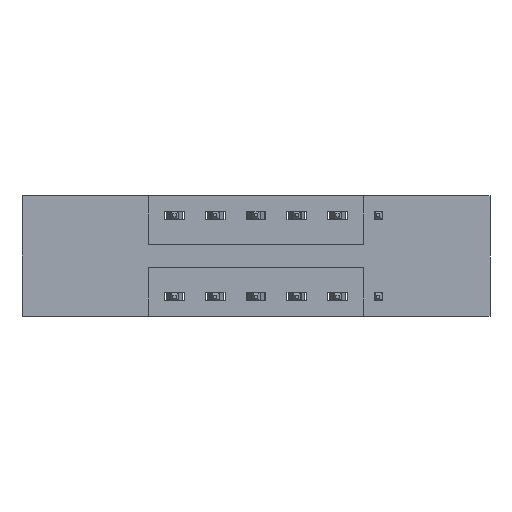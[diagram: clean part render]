
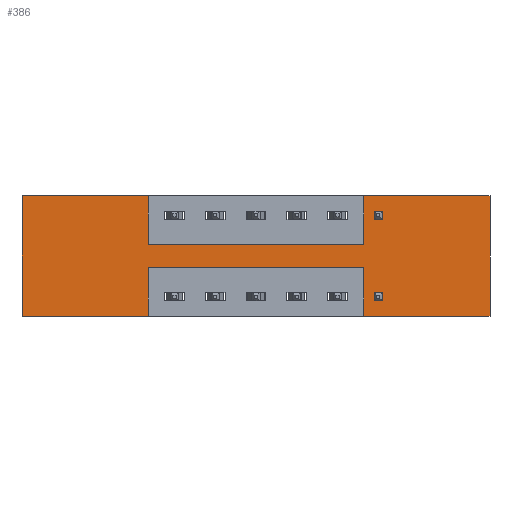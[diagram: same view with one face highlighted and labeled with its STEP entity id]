
A CAD part, front view. The second image highlights one B-rep face of the part: STEP entity #386.
In plain terms, the highlighted planar face has unit normal (0, -1, 0).
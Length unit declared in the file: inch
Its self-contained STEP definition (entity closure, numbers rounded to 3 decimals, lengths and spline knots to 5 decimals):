
#51 = CARTESIAN_POINT ( 'NONE',  ( 0., 0., 0. ) ) ;
#54 = LINE ( 'NONE', #3885, #1753 ) ;
#152 = DIRECTION ( 'NONE',  ( 1., 0., 0. ) ) ;
#193 = CARTESIAN_POINT ( 'NONE',  ( 1.0475, 0., 0. ) ) ;
#250 = VERTEX_POINT ( 'NONE', #798 ) ;
#353 = EDGE_CURVE ( 'NONE', #8071, #6686, #5469, .T. ) ;
#386 = ADVANCED_FACE ( 'NONE', ( #6793 ), #2985, .T. ) ;
#467 = DIRECTION ( 'NONE',  ( 0., -1., 0. ) ) ;
#502 = DIRECTION ( 'NONE',  ( 1., 0., 0. ) ) ;
#661 = CARTESIAN_POINT ( 'NONE',  ( 0., 0., 0. ) ) ;
#690 = VECTOR ( 'NONE', #152, 39.37008 ) ;
#798 = CARTESIAN_POINT ( 'NONE',  ( 0., 0., 0. ) ) ;
#799 = VERTEX_POINT ( 'NONE', #7419 ) ;
#816 = ORIENTED_EDGE ( 'NONE', *, *, #2270, .F. ) ;
#901 = VECTOR ( 'NONE', #8348, 39.37008 ) ;
#942 = VECTOR ( 'NONE', #502, 39.37008 ) ;
#1068 = DIRECTION ( 'NONE',  ( -1., 0., 0. ) ) ;
#1138 = CARTESIAN_POINT ( 'NONE',  ( 1.0475, 0., -0.22 ) ) ;
#1282 = LINE ( 'NONE', #661, #942 ) ;
#1291 = LINE ( 'NONE', #51, #901 ) ;
#1315 = AXIS2_PLACEMENT_3D ( 'NONE', #4908, #467, #3642 ) ;
#1348 = VERTEX_POINT ( 'NONE', #2569 ) ;
#1357 = VERTEX_POINT ( 'NONE', #3238 ) ;
#1665 = LINE ( 'NONE', #4821, #6611 ) ;
#1753 = VECTOR ( 'NONE', #4112, 39.37008 ) ;
#1764 = EDGE_CURVE ( 'NONE', #4762, #2264, #6546, .T. ) ;
#1775 = ORIENTED_EDGE ( 'NONE', *, *, #7255, .F. ) ;
#1805 = DIRECTION ( 'NONE',  ( 0., 0., 1. ) ) ;
#2031 = DIRECTION ( 'NONE',  ( 0., 0., -1. ) ) ;
#2061 = EDGE_CURVE ( 'NONE', #2651, #250, #2506, .T. ) ;
#2093 = DIRECTION ( 'NONE',  ( 0., 0., 1. ) ) ;
#2256 = ORIENTED_EDGE ( 'NONE', *, *, #7544, .F. ) ;
#2264 = VERTEX_POINT ( 'NONE', #7467 ) ;
#2270 = EDGE_CURVE ( 'NONE', #799, #2651, #8138, .T. ) ;
#2292 = LINE ( 'NONE', #6685, #7977 ) ;
#2310 = ORIENTED_EDGE ( 'NONE', *, *, #2061, .F. ) ;
#2506 = LINE ( 'NONE', #8345, #3265 ) ;
#2532 = VECTOR ( 'NONE', #8082, 39.37008 ) ;
#2569 = CARTESIAN_POINT ( 'NONE',  ( 0.3875, 0., -0.22 ) ) ;
#2651 = VERTEX_POINT ( 'NONE', #5196 ) ;
#2677 = LINE ( 'NONE', #5175, #8046 ) ;
#2882 = EDGE_CURVE ( 'NONE', #6908, #6775, #8292, .T. ) ;
#2985 = PLANE ( 'NONE',  #1315 ) ;
#3027 = ORIENTED_EDGE ( 'NONE', *, *, #3664, .F. ) ;
#3066 = ORIENTED_EDGE ( 'NONE', *, *, #3914, .F. ) ;
#3238 = CARTESIAN_POINT ( 'NONE',  ( 0.3875, 0., -0.15 ) ) ;
#3265 = VECTOR ( 'NONE', #3299, 39.37008 ) ;
#3271 = EDGE_CURVE ( 'NONE', #1357, #4762, #3615, .T. ) ;
#3299 = DIRECTION ( 'NONE',  ( 0., 0., 1. ) ) ;
#3323 = CARTESIAN_POINT ( 'NONE',  ( 1.435, 0., -0.37 ) ) ;
#3566 = EDGE_CURVE ( 'NONE', #4511, #1357, #54, .T. ) ;
#3615 = LINE ( 'NONE', #4597, #690 ) ;
#3642 = DIRECTION ( 'NONE',  ( 0., 0., -1. ) ) ;
#3664 = EDGE_CURVE ( 'NONE', #250, #4511, #1282, .T. ) ;
#3788 = CARTESIAN_POINT ( 'NONE',  ( 1.435, 0., 0. ) ) ;
#3800 = VECTOR ( 'NONE', #2093, 39.37008 ) ;
#3885 = CARTESIAN_POINT ( 'NONE',  ( 0.3875, 0., 0. ) ) ;
#3914 = EDGE_CURVE ( 'NONE', #6686, #6908, #1665, .T. ) ;
#4021 = ORIENTED_EDGE ( 'NONE', *, *, #1764, .F. ) ;
#4085 = CARTESIAN_POINT ( 'NONE',  ( 1.0475, 0., -0.15 ) ) ;
#4112 = DIRECTION ( 'NONE',  ( 0., 0., -1. ) ) ;
#4502 = ORIENTED_EDGE ( 'NONE', *, *, #2882, .F. ) ;
#4511 = VERTEX_POINT ( 'NONE', #5579 ) ;
#4597 = CARTESIAN_POINT ( 'NONE',  ( 0.3875, 0., -0.15 ) ) ;
#4709 = ORIENTED_EDGE ( 'NONE', *, *, #3566, .F. ) ;
#4762 = VERTEX_POINT ( 'NONE', #4085 ) ;
#4821 = CARTESIAN_POINT ( 'NONE',  ( 0., 0., -0.37 ) ) ;
#4908 = CARTESIAN_POINT ( 'NONE',  ( 0., 0., -0.37 ) ) ;
#5058 = CARTESIAN_POINT ( 'NONE',  ( 1.0475, 0., -0.37 ) ) ;
#5175 = CARTESIAN_POINT ( 'NONE',  ( 0.3875, 0., -0.37 ) ) ;
#5196 = CARTESIAN_POINT ( 'NONE',  ( 0., 0., -0.37 ) ) ;
#5362 = EDGE_CURVE ( 'NONE', #6775, #1348, #2292, .T. ) ;
#5469 = LINE ( 'NONE', #8132, #2532 ) ;
#5579 = CARTESIAN_POINT ( 'NONE',  ( 0.3875, 0., 0. ) ) ;
#6191 = EDGE_LOOP ( 'NONE', ( #2256, #7486, #4502, #3066, #6756, #1775, #4021, #6309, #4709, #3027, #2310, #816 ) ) ;
#6309 = ORIENTED_EDGE ( 'NONE', *, *, #3271, .F. ) ;
#6546 = LINE ( 'NONE', #193, #3800 ) ;
#6611 = VECTOR ( 'NONE', #1068, 39.37008 ) ;
#6685 = CARTESIAN_POINT ( 'NONE',  ( 0.3875, 0., -0.22 ) ) ;
#6686 = VERTEX_POINT ( 'NONE', #3323 ) ;
#6744 = DIRECTION ( 'NONE',  ( -1., 0., 0. ) ) ;
#6756 = ORIENTED_EDGE ( 'NONE', *, *, #353, .F. ) ;
#6775 = VERTEX_POINT ( 'NONE', #1138 ) ;
#6793 = FACE_OUTER_BOUND ( 'NONE', #6191, .T. ) ;
#6908 = VERTEX_POINT ( 'NONE', #8320 ) ;
#7181 = VECTOR ( 'NONE', #6744, 39.37008 ) ;
#7255 = EDGE_CURVE ( 'NONE', #2264, #8071, #1291, .T. ) ;
#7368 = CARTESIAN_POINT ( 'NONE',  ( 0., 0., -0.37 ) ) ;
#7419 = CARTESIAN_POINT ( 'NONE',  ( 0.3875, 0., -0.37 ) ) ;
#7450 = DIRECTION ( 'NONE',  ( -1., 0., 0. ) ) ;
#7467 = CARTESIAN_POINT ( 'NONE',  ( 1.0475, 0., 0. ) ) ;
#7486 = ORIENTED_EDGE ( 'NONE', *, *, #5362, .F. ) ;
#7544 = EDGE_CURVE ( 'NONE', #1348, #799, #2677, .T. ) ;
#7823 = VECTOR ( 'NONE', #1805, 39.37008 ) ;
#7977 = VECTOR ( 'NONE', #7450, 39.37008 ) ;
#8046 = VECTOR ( 'NONE', #2031, 39.37008 ) ;
#8071 = VERTEX_POINT ( 'NONE', #3788 ) ;
#8082 = DIRECTION ( 'NONE',  ( 0., 0., -1. ) ) ;
#8132 = CARTESIAN_POINT ( 'NONE',  ( 1.435, 0., 0. ) ) ;
#8138 = LINE ( 'NONE', #7368, #7181 ) ;
#8292 = LINE ( 'NONE', #5058, #7823 ) ;
#8320 = CARTESIAN_POINT ( 'NONE',  ( 1.0475, 0., -0.37 ) ) ;
#8345 = CARTESIAN_POINT ( 'NONE',  ( 0., 0., 0. ) ) ;
#8348 = DIRECTION ( 'NONE',  ( 1., 0., 0. ) ) ;
